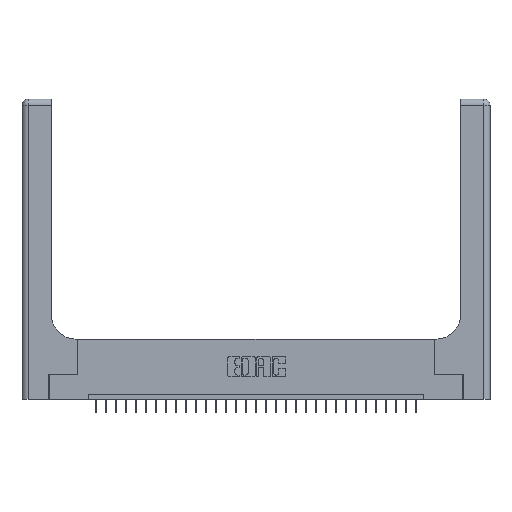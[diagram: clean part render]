
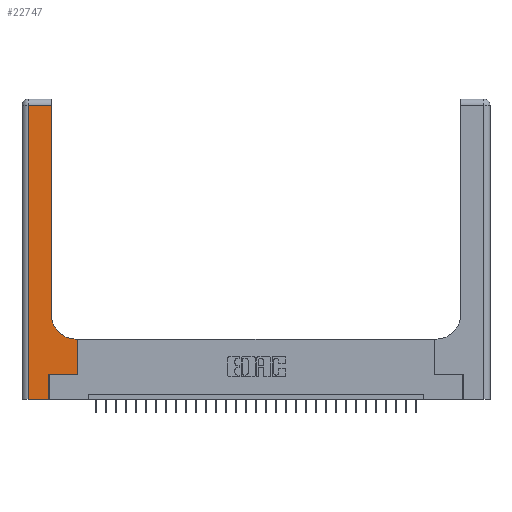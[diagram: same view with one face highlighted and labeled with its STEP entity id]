
A CAD part, top view. The second image highlights one B-rep face of the part: STEP entity #22747.
In plain terms, the highlighted planar face has unit normal (0, 0, 1).
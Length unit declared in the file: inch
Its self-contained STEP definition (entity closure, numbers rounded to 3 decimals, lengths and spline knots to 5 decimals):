
#425 = CARTESIAN_POINT ( 'NONE',  ( 0.269, 0., 0.37 ) ) ;
#679 = EDGE_CURVE ( 'NONE', #26357, #26923, #17057, .T. ) ;
#1419 = ORIENTED_EDGE ( 'NONE', *, *, #679, .T. ) ;
#1593 = CARTESIAN_POINT ( 'NONE',  ( 0.269, 0.25, 0.37 ) ) ;
#2306 = DIRECTION ( 'NONE',  ( -1., 0., 0. ) ) ;
#2715 = DIRECTION ( 'NONE',  ( 1., 0., 0. ) ) ;
#2951 = DIRECTION ( 'NONE',  ( 0., 0., -1. ) ) ;
#3471 = VERTEX_POINT ( 'NONE', #425 ) ;
#3690 = EDGE_CURVE ( 'NONE', #3471, #10265, #23342, .T. ) ;
#3864 = DIRECTION ( 'NONE',  ( 0., 1., 0. ) ) ;
#4420 = FACE_OUTER_BOUND ( 'NONE', #25230, .T. ) ;
#4606 = VECTOR ( 'NONE', #2715, 39.37008 ) ;
#5003 = EDGE_CURVE ( 'NONE', #30583, #3471, #17760, .T. ) ;
#5163 = ORIENTED_EDGE ( 'NONE', *, *, #5003, .T. ) ;
#6227 = CARTESIAN_POINT ( 'NONE',  ( 0.5585, 0.6, 0.37 ) ) ;
#6508 = CARTESIAN_POINT ( 'NONE',  ( 0., 3., 0.37 ) ) ;
#6802 = EDGE_CURVE ( 'NONE', #29190, #24956, #18960, .T. ) ;
#7189 = CARTESIAN_POINT ( 'NONE',  ( 0.06, 0., 0.37 ) ) ;
#7573 = CARTESIAN_POINT ( 'NONE',  ( 0., 2.94, 0.37 ) ) ;
#8124 = CARTESIAN_POINT ( 'NONE',  ( 0., 0., 0.37 ) ) ;
#10004 = VECTOR ( 'NONE', #20348, 39.37008 ) ;
#10265 = VERTEX_POINT ( 'NONE', #30246 ) ;
#10340 = ORIENTED_EDGE ( 'NONE', *, *, #3690, .T. ) ;
#10406 = DIRECTION ( 'NONE',  ( 1., 0., 0. ) ) ;
#10630 = CARTESIAN_POINT ( 'NONE',  ( 0.06, 2.94, 0.37 ) ) ;
#10797 = LINE ( 'NONE', #1593, #29099 ) ;
#10997 = EDGE_CURVE ( 'NONE', #21310, #30583, #22884, .T. ) ;
#11441 = ORIENTED_EDGE ( 'NONE', *, *, #23280, .T. ) ;
#11817 = ORIENTED_EDGE ( 'NONE', *, *, #6802, .T. ) ;
#12042 = VECTOR ( 'NONE', #17203, 39.37008 ) ;
#13032 = AXIS2_PLACEMENT_3D ( 'NONE', #6508, #18666, #13771 ) ;
#13437 = EDGE_CURVE ( 'NONE', #10265, #29190, #10797, .T. ) ;
#13771 = DIRECTION ( 'NONE',  ( -1., 0., 0. ) ) ;
#14355 = CARTESIAN_POINT ( 'NONE',  ( 0.2915, 2.94, 0.37 ) ) ;
#14488 = CARTESIAN_POINT ( 'NONE',  ( 0.2915, 0.6, 0.37 ) ) ;
#15684 = DIRECTION ( 'NONE',  ( 1., 0., 0. ) ) ;
#16422 = DIRECTION ( 'NONE',  ( 0., 1., 0. ) ) ;
#17057 = CIRCLE ( 'NONE', #28216, 0.25 ) ;
#17203 = DIRECTION ( 'NONE',  ( -1., 0., 0. ) ) ;
#17760 = LINE ( 'NONE', #8124, #4606 ) ;
#17954 = DIRECTION ( 'NONE',  ( 0., -1., 0. ) ) ;
#18326 = CARTESIAN_POINT ( 'NONE',  ( 0.2915, 0.85, 0.37 ) ) ;
#18666 = DIRECTION ( 'NONE',  ( 0., 0., -1. ) ) ;
#18727 = VERTEX_POINT ( 'NONE', #14355 ) ;
#18751 = ORIENTED_EDGE ( 'NONE', *, *, #23767, .T. ) ;
#18960 = LINE ( 'NONE', #30861, #25931 ) ;
#20142 = EDGE_CURVE ( 'NONE', #24956, #26357, #24167, .T. ) ;
#20348 = DIRECTION ( 'NONE',  ( 0., 1., 0. ) ) ;
#20817 = VECTOR ( 'NONE', #3864, 39.37008 ) ;
#21310 = VERTEX_POINT ( 'NONE', #10630 ) ;
#22105 = VECTOR ( 'NONE', #2306, 39.37008 ) ;
#22747 = ADVANCED_FACE ( 'NONE', ( #4420 ), #28486, .F. ) ;
#22884 = LINE ( 'NONE', #29691, #25651 ) ;
#23043 = CARTESIAN_POINT ( 'NONE',  ( 0.2915, 3., 0.37 ) ) ;
#23280 = EDGE_CURVE ( 'NONE', #26923, #18727, #30175, .T. ) ;
#23342 = LINE ( 'NONE', #25543, #20817 ) ;
#23767 = EDGE_CURVE ( 'NONE', #18727, #21310, #29251, .T. ) ;
#24167 = LINE ( 'NONE', #14488, #22105 ) ;
#24811 = CARTESIAN_POINT ( 'NONE',  ( 0.5415, 0.85, 0.37 ) ) ;
#24956 = VERTEX_POINT ( 'NONE', #6227 ) ;
#25230 = EDGE_LOOP ( 'NONE', ( #11441, #18751, #30866, #5163, #10340, #30157, #11817, #25733, #1419 ) ) ;
#25543 = CARTESIAN_POINT ( 'NONE',  ( 0.269, 0., 0.37 ) ) ;
#25651 = VECTOR ( 'NONE', #17954, 39.37008 ) ;
#25733 = ORIENTED_EDGE ( 'NONE', *, *, #20142, .T. ) ;
#25931 = VECTOR ( 'NONE', #16422, 39.37008 ) ;
#26357 = VERTEX_POINT ( 'NONE', #31048 ) ;
#26923 = VERTEX_POINT ( 'NONE', #18326 ) ;
#27476 = CARTESIAN_POINT ( 'NONE',  ( 0.5585, 0.25, 0.37 ) ) ;
#28216 = AXIS2_PLACEMENT_3D ( 'NONE', #24811, #2951, #10406 ) ;
#28486 = PLANE ( 'NONE',  #13032 ) ;
#29099 = VECTOR ( 'NONE', #15684, 39.37008 ) ;
#29190 = VERTEX_POINT ( 'NONE', #27476 ) ;
#29251 = LINE ( 'NONE', #7573, #12042 ) ;
#29691 = CARTESIAN_POINT ( 'NONE',  ( 0.06, 3., 0.37 ) ) ;
#30157 = ORIENTED_EDGE ( 'NONE', *, *, #13437, .T. ) ;
#30175 = LINE ( 'NONE', #23043, #10004 ) ;
#30246 = CARTESIAN_POINT ( 'NONE',  ( 0.269, 0.25, 0.37 ) ) ;
#30583 = VERTEX_POINT ( 'NONE', #7189 ) ;
#30861 = CARTESIAN_POINT ( 'NONE',  ( 0.5585, 0.25, 0.37 ) ) ;
#30866 = ORIENTED_EDGE ( 'NONE', *, *, #10997, .T. ) ;
#31048 = CARTESIAN_POINT ( 'NONE',  ( 0.5415, 0.6, 0.37 ) ) ;
